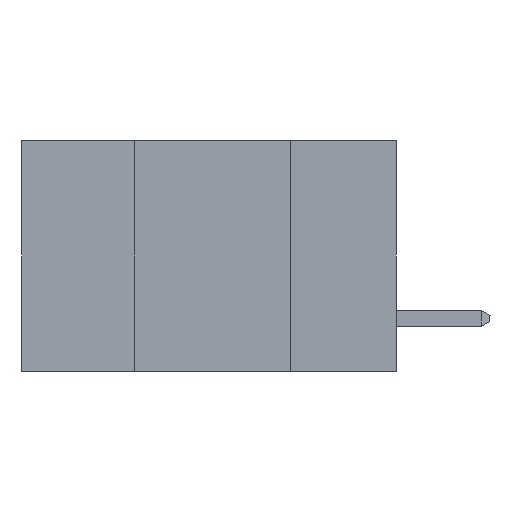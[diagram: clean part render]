
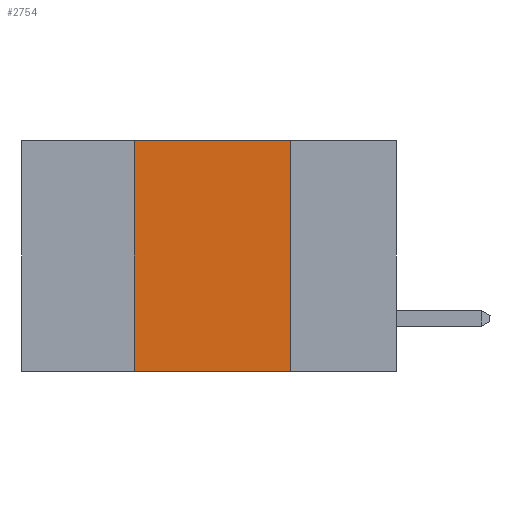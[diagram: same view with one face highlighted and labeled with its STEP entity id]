
A CAD part, left-side view. The second image highlights one B-rep face of the part: STEP entity #2754.
In plain terms, the highlighted planar face has unit normal (-1, 0, 0).
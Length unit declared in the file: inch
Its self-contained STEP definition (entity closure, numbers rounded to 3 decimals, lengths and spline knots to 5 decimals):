
#35 = DIRECTION ( 'NONE',  ( 1., 0., 0. ) ) ;
#148 = DIRECTION ( 'NONE',  ( 0., -1., 0. ) ) ;
#477 = CARTESIAN_POINT ( 'NONE',  ( 0., 0.17, -0.37 ) ) ;
#1209 = DIRECTION ( 'NONE',  ( 0., 0., -1. ) ) ;
#1336 = AXIS2_PLACEMENT_3D ( 'NONE', #4536, #35, #1209 ) ;
#1522 = CARTESIAN_POINT ( 'NONE',  ( 0., 0.6, 0. ) ) ;
#1589 = VERTEX_POINT ( 'NONE', #8005 ) ;
#1907 = EDGE_CURVE ( 'NONE', #6220, #3203, #8579, .T. ) ;
#2008 = VECTOR ( 'NONE', #4374, 39.37008 ) ;
#2445 = ORIENTED_EDGE ( 'NONE', *, *, #1907, .F. ) ;
#2754 = ADVANCED_FACE ( 'NONE', ( #9609 ), #13074, .F. ) ;
#3076 = EDGE_LOOP ( 'NONE', ( #4620, #9042, #2445, #3640 ) ) ;
#3203 = VERTEX_POINT ( 'NONE', #8130 ) ;
#3640 = ORIENTED_EDGE ( 'NONE', *, *, #4213, .T. ) ;
#4213 = EDGE_CURVE ( 'NONE', #6220, #8823, #11029, .T. ) ;
#4374 = DIRECTION ( 'NONE',  ( 0., 0., -1. ) ) ;
#4536 = CARTESIAN_POINT ( 'NONE',  ( 0., 0.6, 0. ) ) ;
#4620 = ORIENTED_EDGE ( 'NONE', *, *, #6032, .F. ) ;
#4637 = CARTESIAN_POINT ( 'NONE',  ( 0., 0.42, -0.37 ) ) ;
#5417 = LINE ( 'NONE', #10398, #2008 ) ;
#5603 = VECTOR ( 'NONE', #9713, 39.37008 ) ;
#6032 = EDGE_CURVE ( 'NONE', #1589, #8823, #5417, .T. ) ;
#6220 = VERTEX_POINT ( 'NONE', #9941 ) ;
#6228 = VECTOR ( 'NONE', #8025, 39.37008 ) ;
#8005 = CARTESIAN_POINT ( 'NONE',  ( 0., 0.17, 0. ) ) ;
#8025 = DIRECTION ( 'NONE',  ( 0., -1., 0. ) ) ;
#8130 = CARTESIAN_POINT ( 'NONE',  ( 0., 0.42, 0. ) ) ;
#8333 = VECTOR ( 'NONE', #148, 39.37008 ) ;
#8579 = LINE ( 'NONE', #4637, #5603 ) ;
#8740 = LINE ( 'NONE', #1522, #8333 ) ;
#8823 = VERTEX_POINT ( 'NONE', #477 ) ;
#9042 = ORIENTED_EDGE ( 'NONE', *, *, #11206, .F. ) ;
#9609 = FACE_OUTER_BOUND ( 'NONE', #3076, .T. ) ;
#9713 = DIRECTION ( 'NONE',  ( 0., 0., 1. ) ) ;
#9941 = CARTESIAN_POINT ( 'NONE',  ( 0., 0.42, -0.37 ) ) ;
#10398 = CARTESIAN_POINT ( 'NONE',  ( 0., 0.17, -0.37 ) ) ;
#11029 = LINE ( 'NONE', #11253, #6228 ) ;
#11206 = EDGE_CURVE ( 'NONE', #3203, #1589, #8740, .T. ) ;
#11253 = CARTESIAN_POINT ( 'NONE',  ( 0., 0.6, -0.37 ) ) ;
#13074 = PLANE ( 'NONE',  #1336 ) ;
